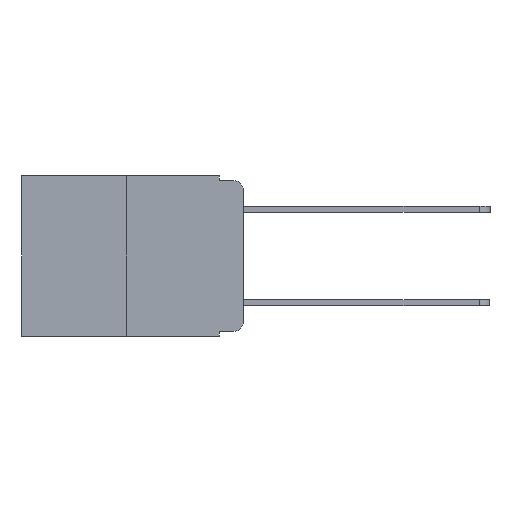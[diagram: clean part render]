
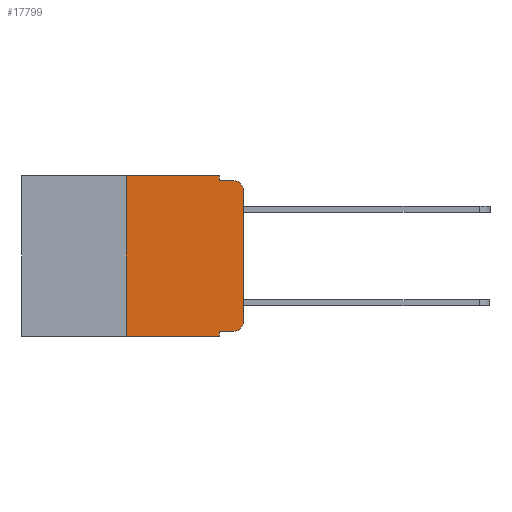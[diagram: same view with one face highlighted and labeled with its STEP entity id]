
A CAD part, left-side view. The second image highlights one B-rep face of the part: STEP entity #17799.
In plain terms, the highlighted planar face has unit normal (-1, 0, 0).
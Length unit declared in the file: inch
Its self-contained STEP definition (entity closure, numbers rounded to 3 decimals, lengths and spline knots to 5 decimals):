
#314 = ORIENTED_EDGE ( 'NONE', *, *, #21635, .F. ) ;
#482 = EDGE_CURVE ( 'NONE', #3289, #21065, #10874, .T. ) ;
#541 = CARTESIAN_POINT ( 'NONE',  ( 0., 0.051, 0. ) ) ;
#644 = CARTESIAN_POINT ( 'NONE',  ( 0., 0.051, -0.01 ) ) ;
#937 = VERTEX_POINT ( 'NONE', #14799 ) ;
#2364 = LINE ( 'NONE', #24924, #22860 ) ;
#2378 = AXIS2_PLACEMENT_3D ( 'NONE', #11353, #24765, #13281 ) ;
#2887 = CARTESIAN_POINT ( 'NONE',  ( 0., 0., 0. ) ) ;
#3179 = VECTOR ( 'NONE', #21084, 39.37008 ) ;
#3289 = VERTEX_POINT ( 'NONE', #3969 ) ;
#3753 = DIRECTION ( 'NONE',  ( 0., -1., 0. ) ) ;
#3815 = CARTESIAN_POINT ( 'NONE',  ( 0., 0.051, -0.333 ) ) ;
#3969 = CARTESIAN_POINT ( 'NONE',  ( 0., 0.25, 0. ) ) ;
#4027 = VERTEX_POINT ( 'NONE', #11924 ) ;
#4204 = DIRECTION ( 'NONE',  ( 0., -1., 0. ) ) ;
#4295 = CARTESIAN_POINT ( 'NONE',  ( 0., 0., -0.313 ) ) ;
#4455 = VECTOR ( 'NONE', #10111, 39.37008 ) ;
#4586 = ORIENTED_EDGE ( 'NONE', *, *, #8055, .T. ) ;
#5558 = CARTESIAN_POINT ( 'NONE',  ( 0., 0.473, 0. ) ) ;
#5725 = CARTESIAN_POINT ( 'NONE',  ( 0., 0.051, 0. ) ) ;
#5838 = LINE ( 'NONE', #2887, #16093 ) ;
#6239 = CARTESIAN_POINT ( 'NONE',  ( 0., 0.051, -0.01 ) ) ;
#6986 = VERTEX_POINT ( 'NONE', #12976 ) ;
#7393 = LINE ( 'NONE', #3815, #12468 ) ;
#7426 = VECTOR ( 'NONE', #12144, 39.37008 ) ;
#8016 = LINE ( 'NONE', #23636, #7426 ) ;
#8055 = EDGE_CURVE ( 'NONE', #9034, #8339, #23055, .T. ) ;
#8339 = VERTEX_POINT ( 'NONE', #4295 ) ;
#9034 = VERTEX_POINT ( 'NONE', #23235 ) ;
#9450 = VECTOR ( 'NONE', #4204, 39.37008 ) ;
#9571 = EDGE_CURVE ( 'NONE', #17616, #9034, #7393, .T. ) ;
#10111 = DIRECTION ( 'NONE',  ( 0., 0., 1. ) ) ;
#10412 = CARTESIAN_POINT ( 'NONE',  ( 0., 0., -0.03 ) ) ;
#10572 = DIRECTION ( 'NONE',  ( 0., 0., 1. ) ) ;
#10874 = LINE ( 'NONE', #5558, #16020 ) ;
#11007 = DIRECTION ( 'NONE',  ( 0., 0., -1. ) ) ;
#11126 = CARTESIAN_POINT ( 'NONE',  ( 0., 0.02, -0.313 ) ) ;
#11353 = CARTESIAN_POINT ( 'NONE',  ( 0., 0.02, -0.03 ) ) ;
#11924 = CARTESIAN_POINT ( 'NONE',  ( 0., 0.25, -0.343 ) ) ;
#12043 = ORIENTED_EDGE ( 'NONE', *, *, #22098, .F. ) ;
#12144 = DIRECTION ( 'NONE',  ( 0., 0., -1. ) ) ;
#12335 = EDGE_CURVE ( 'NONE', #22887, #937, #19689, .T. ) ;
#12338 = CARTESIAN_POINT ( 'NONE',  ( 0., 0.051, -0.333 ) ) ;
#12468 = VECTOR ( 'NONE', #24899, 39.37008 ) ;
#12513 = ORIENTED_EDGE ( 'NONE', *, *, #19745, .T. ) ;
#12518 = EDGE_CURVE ( 'NONE', #8339, #24154, #5838, .T. ) ;
#12976 = CARTESIAN_POINT ( 'NONE',  ( 0., 0.051, -0.343 ) ) ;
#13059 = DIRECTION ( 'NONE',  ( 0., 0., -1. ) ) ;
#13281 = DIRECTION ( 'NONE',  ( 0., 0., -1. ) ) ;
#13515 = EDGE_LOOP ( 'NONE', ( #14440, #15069, #19036, #17312, #15825, #314, #12513, #12043, #20806, #4586 ) ) ;
#13690 = EDGE_CURVE ( 'NONE', #24154, #937, #23379, .T. ) ;
#14440 = ORIENTED_EDGE ( 'NONE', *, *, #12518, .T. ) ;
#14696 = EDGE_CURVE ( 'NONE', #21065, #22887, #8016, .T. ) ;
#14799 = CARTESIAN_POINT ( 'NONE',  ( 0., 0.02, -0.01 ) ) ;
#14816 = CARTESIAN_POINT ( 'NONE',  ( 0., 0.473, 0. ) ) ;
#14864 = FACE_OUTER_BOUND ( 'NONE', #13515, .T. ) ;
#15069 = ORIENTED_EDGE ( 'NONE', *, *, #13690, .T. ) ;
#15825 = ORIENTED_EDGE ( 'NONE', *, *, #482, .F. ) ;
#16020 = VECTOR ( 'NONE', #23439, 39.37008 ) ;
#16093 = VECTOR ( 'NONE', #10572, 39.37008 ) ;
#17312 = ORIENTED_EDGE ( 'NONE', *, *, #14696, .F. ) ;
#17616 = VERTEX_POINT ( 'NONE', #12338 ) ;
#17799 = ADVANCED_FACE ( 'NONE', ( #14864 ), #20582, .F. ) ;
#19036 = ORIENTED_EDGE ( 'NONE', *, *, #12335, .F. ) ;
#19206 = LINE ( 'NONE', #23519, #4455 ) ;
#19689 = LINE ( 'NONE', #6239, #9450 ) ;
#19745 = EDGE_CURVE ( 'NONE', #4027, #6986, #2364, .T. ) ;
#19786 = AXIS2_PLACEMENT_3D ( 'NONE', #14816, #22493, #11007 ) ;
#20582 = PLANE ( 'NONE',  #19786 ) ;
#20806 = ORIENTED_EDGE ( 'NONE', *, *, #9571, .T. ) ;
#21065 = VERTEX_POINT ( 'NONE', #541 ) ;
#21084 = DIRECTION ( 'NONE',  ( 0., 0., -1. ) ) ;
#21635 = EDGE_CURVE ( 'NONE', #4027, #3289, #19206, .T. ) ;
#22098 = EDGE_CURVE ( 'NONE', #17616, #6986, #24244, .T. ) ;
#22493 = DIRECTION ( 'NONE',  ( 1., 0., 0. ) ) ;
#22860 = VECTOR ( 'NONE', #3753, 39.37008 ) ;
#22887 = VERTEX_POINT ( 'NONE', #644 ) ;
#23055 = CIRCLE ( 'NONE', #24415, 0.02 ) ;
#23235 = CARTESIAN_POINT ( 'NONE',  ( 0., 0.02, -0.333 ) ) ;
#23379 = CIRCLE ( 'NONE', #2378, 0.02 ) ;
#23439 = DIRECTION ( 'NONE',  ( 0., -1., 0. ) ) ;
#23519 = CARTESIAN_POINT ( 'NONE',  ( 0., 0.25, 0. ) ) ;
#23636 = CARTESIAN_POINT ( 'NONE',  ( 0., 0.051, 0. ) ) ;
#24154 = VERTEX_POINT ( 'NONE', #10412 ) ;
#24244 = LINE ( 'NONE', #5725, #3179 ) ;
#24415 = AXIS2_PLACEMENT_3D ( 'NONE', #11126, #24549, #13059 ) ;
#24549 = DIRECTION ( 'NONE',  ( -1., 0., 0. ) ) ;
#24765 = DIRECTION ( 'NONE',  ( -1., 0., 0. ) ) ;
#24899 = DIRECTION ( 'NONE',  ( 0., -1., 0. ) ) ;
#24924 = CARTESIAN_POINT ( 'NONE',  ( 0., 0.473, -0.343 ) ) ;
